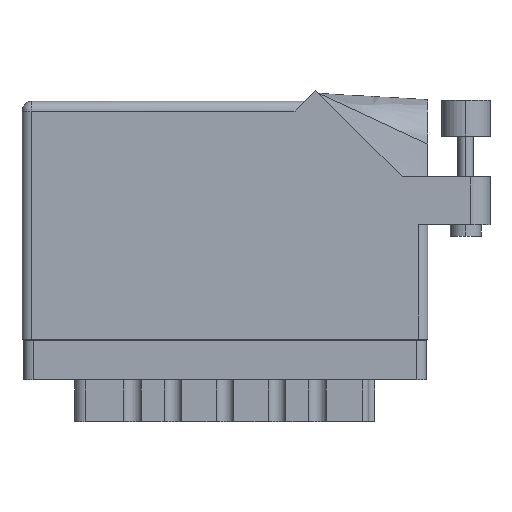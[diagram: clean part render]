
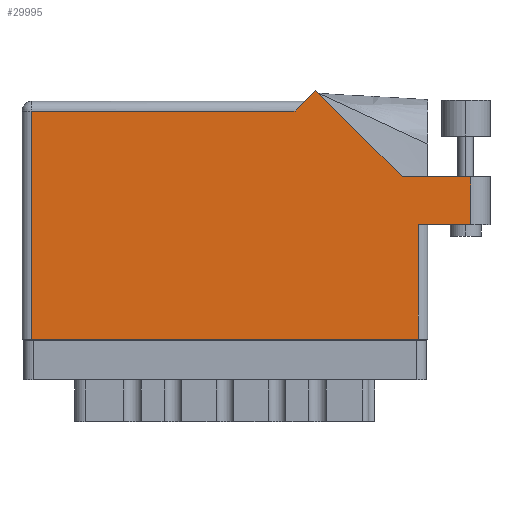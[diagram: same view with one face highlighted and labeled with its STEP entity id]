
A CAD part, front view. The second image highlights one B-rep face of the part: STEP entity #29995.
In plain terms, the highlighted face is planar.
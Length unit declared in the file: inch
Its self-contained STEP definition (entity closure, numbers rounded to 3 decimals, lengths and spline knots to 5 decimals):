
#50 = EDGE_CURVE ( 'NONE', #861, #7636, #42024, .T. ) ;
#249 = VECTOR ( 'NONE', #8131, 39.37008 ) ;
#861 = VERTEX_POINT ( 'NONE', #42348 ) ;
#1576 = DIRECTION ( 'NONE',  ( -0.707, -0.707, 0. ) ) ;
#1802 = CARTESIAN_POINT ( 'NONE',  ( 0.062, 1.468, 0. ) ) ;
#2515 = LINE ( 'NONE', #19413, #9093 ) ;
#3708 = DIRECTION ( 'NONE',  ( -1., 0., 0. ) ) ;
#4006 = CARTESIAN_POINT ( 'NONE',  ( 2.887, 0.737, 0. ) ) ;
#4476 = CARTESIAN_POINT ( 'NONE',  ( 2.44642, 1.044, 0. ) ) ;
#5727 = FACE_OUTER_BOUND ( 'NONE', #40813, .T. ) ;
#6197 = VERTEX_POINT ( 'NONE', #7866 ) ;
#6866 = CARTESIAN_POINT ( 'NONE',  ( 3.012, 1.044, 0. ) ) ;
#7542 = CARTESIAN_POINT ( 'NONE',  ( 0., 0., 0. ) ) ;
#7636 = VERTEX_POINT ( 'NONE', #4476 ) ;
#7866 = CARTESIAN_POINT ( 'NONE',  ( 1.88971, 1.60071, 0. ) ) ;
#8131 = DIRECTION ( 'NONE',  ( 0., 1., 0. ) ) ;
#8882 = EDGE_CURVE ( 'NONE', #7636, #6197, #21675, .T. ) ;
#9093 = VECTOR ( 'NONE', #11384, 39.37008 ) ;
#9491 = VECTOR ( 'NONE', #32491, 39.37008 ) ;
#10114 = LINE ( 'NONE', #27763, #26837 ) ;
#10145 = DIRECTION ( 'NONE',  ( -0.707, 0.707, 0. ) ) ;
#11092 = ORIENTED_EDGE ( 'NONE', *, *, #30577, .T. ) ;
#11231 = VERTEX_POINT ( 'NONE', #1802 ) ;
#11384 = DIRECTION ( 'NONE',  ( -1., 0., 0. ) ) ;
#11830 = CARTESIAN_POINT ( 'NONE',  ( 0.062, 0., 0. ) ) ;
#13136 = CARTESIAN_POINT ( 'NONE',  ( 2.887, 1.044, 0. ) ) ;
#13839 = CARTESIAN_POINT ( 'NONE',  ( 2.44642, 1.044, 0. ) ) ;
#14419 = ORIENTED_EDGE ( 'NONE', *, *, #50, .T. ) ;
#15125 = VERTEX_POINT ( 'NONE', #11830 ) ;
#15135 = EDGE_CURVE ( 'NONE', #42957, #32394, #38885, .T. ) ;
#16830 = CARTESIAN_POINT ( 'NONE',  ( 1.819, 1.53, 0. ) ) ;
#17448 = AXIS2_PLACEMENT_3D ( 'NONE', #46282, #38274, #3708 ) ;
#19127 = LINE ( 'NONE', #16830, #32270 ) ;
#19413 = CARTESIAN_POINT ( 'NONE',  ( 0., 1.468, 0. ) ) ;
#21675 = LINE ( 'NONE', #13839, #31282 ) ;
#22242 = DIRECTION ( 'NONE',  ( -1., 0., 0. ) ) ;
#23591 = LINE ( 'NONE', #31029, #249 ) ;
#24528 = ORIENTED_EDGE ( 'NONE', *, *, #31430, .T. ) ;
#26232 = LINE ( 'NONE', #13136, #9491 ) ;
#26682 = DIRECTION ( 'NONE',  ( 1., 0., 0. ) ) ;
#26837 = VECTOR ( 'NONE', #47472, 39.37008 ) ;
#27763 = CARTESIAN_POINT ( 'NONE',  ( 0.062, 0., 0. ) ) ;
#29548 = VERTEX_POINT ( 'NONE', #35175 ) ;
#29995 = ADVANCED_FACE ( 'NONE', ( #5727 ), #30605, .F. ) ;
#30127 = EDGE_CURVE ( 'NONE', #15125, #29548, #40955, .T. ) ;
#30577 = EDGE_CURVE ( 'NONE', #29548, #42957, #23591, .T. ) ;
#30605 = PLANE ( 'NONE',  #17448 ) ;
#30808 = VECTOR ( 'NONE', #35605, 39.37008 ) ;
#31029 = CARTESIAN_POINT ( 'NONE',  ( 2.55, 0.737, 0. ) ) ;
#31282 = VECTOR ( 'NONE', #10145, 39.37008 ) ;
#31430 = EDGE_CURVE ( 'NONE', #6197, #43458, #19127, .T. ) ;
#32157 = ORIENTED_EDGE ( 'NONE', *, *, #30127, .T. ) ;
#32270 = VECTOR ( 'NONE', #1576, 39.37008 ) ;
#32394 = VERTEX_POINT ( 'NONE', #4006 ) ;
#32491 = DIRECTION ( 'NONE',  ( 0., 1., 0. ) ) ;
#32542 = ORIENTED_EDGE ( 'NONE', *, *, #8882, .T. ) ;
#35175 = CARTESIAN_POINT ( 'NONE',  ( 2.55, 0., 0. ) ) ;
#35605 = DIRECTION ( 'NONE',  ( 1., 0., 0. ) ) ;
#38274 = DIRECTION ( 'NONE',  ( 0., 0., -1. ) ) ;
#38885 = LINE ( 'NONE', #45725, #43647 ) ;
#39687 = CARTESIAN_POINT ( 'NONE',  ( 1.757, 1.468, 0. ) ) ;
#39692 = EDGE_CURVE ( 'NONE', #43458, #11231, #2515, .T. ) ;
#40713 = ORIENTED_EDGE ( 'NONE', *, *, #15135, .T. ) ;
#40745 = CARTESIAN_POINT ( 'NONE',  ( 2.55, 0.737, 0. ) ) ;
#40813 = EDGE_LOOP ( 'NONE', ( #40713, #44682, #14419, #32542, #24528, #43863, #42515, #32157, #11092 ) ) ;
#40955 = LINE ( 'NONE', #7542, #30808 ) ;
#42024 = LINE ( 'NONE', #6866, #47405 ) ;
#42348 = CARTESIAN_POINT ( 'NONE',  ( 2.887, 1.044, 0. ) ) ;
#42515 = ORIENTED_EDGE ( 'NONE', *, *, #45695, .T. ) ;
#42957 = VERTEX_POINT ( 'NONE', #40745 ) ;
#43458 = VERTEX_POINT ( 'NONE', #39687 ) ;
#43647 = VECTOR ( 'NONE', #26682, 39.37008 ) ;
#43863 = ORIENTED_EDGE ( 'NONE', *, *, #39692, .T. ) ;
#44682 = ORIENTED_EDGE ( 'NONE', *, *, #46810, .T. ) ;
#45695 = EDGE_CURVE ( 'NONE', #11231, #15125, #10114, .T. ) ;
#45725 = CARTESIAN_POINT ( 'NONE',  ( 2.612, 0.737, 0. ) ) ;
#46282 = CARTESIAN_POINT ( 'NONE',  ( 0., 1.53, 0. ) ) ;
#46810 = EDGE_CURVE ( 'NONE', #32394, #861, #26232, .T. ) ;
#47405 = VECTOR ( 'NONE', #22242, 39.37008 ) ;
#47472 = DIRECTION ( 'NONE',  ( 0., -1., 0. ) ) ;
